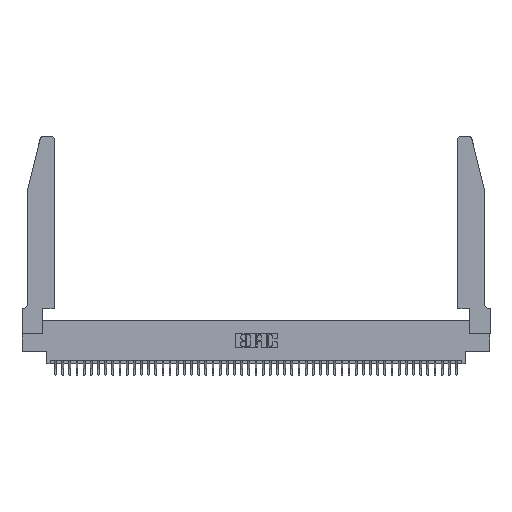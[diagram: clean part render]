
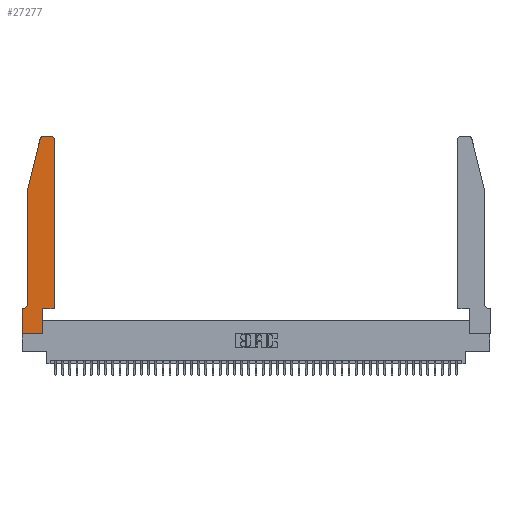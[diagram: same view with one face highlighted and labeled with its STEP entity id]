
A CAD part, top view. The second image highlights one B-rep face of the part: STEP entity #27277.
In plain terms, the highlighted planar face has unit normal (0, 0, 1).
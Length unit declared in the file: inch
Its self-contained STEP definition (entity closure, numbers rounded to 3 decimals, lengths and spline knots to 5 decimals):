
#20 = ORIENTED_EDGE ( 'NONE', *, *, #19385, .T. ) ;
#1429 = CARTESIAN_POINT ( 'NONE',  ( 0.4205, 2.75, 0.37 ) ) ;
#1964 = EDGE_CURVE ( 'NONE', #38628, #4420, #27230, .T. ) ;
#2141 = CARTESIAN_POINT ( 'NONE',  ( 0.4505, 0.35, 0.37 ) ) ;
#2412 = CARTESIAN_POINT ( 'NONE',  ( 0.2865, 0., 0.37 ) ) ;
#2573 = AXIS2_PLACEMENT_3D ( 'NONE', #45537, #16518, #23485 ) ;
#2690 = CARTESIAN_POINT ( 'NONE',  ( 0.0755, 2., 0.37 ) ) ;
#3716 = VECTOR ( 'NONE', #24638, 39.37008 ) ;
#3893 = EDGE_CURVE ( 'NONE', #40289, #14073, #43181, .T. ) ;
#4172 = CARTESIAN_POINT ( 'NONE',  ( 0.4505, 2.72, 0.37 ) ) ;
#4420 = VERTEX_POINT ( 'NONE', #40734 ) ;
#4967 = DIRECTION ( 'NONE',  ( 1., 0., 0. ) ) ;
#5245 = DIRECTION ( 'NONE',  ( 0., -1., 0. ) ) ;
#5766 = LINE ( 'NONE', #35948, #44447 ) ;
#6378 = ORIENTED_EDGE ( 'NONE', *, *, #39761, .T. ) ;
#6532 = LINE ( 'NONE', #11132, #37181 ) ;
#7448 = CARTESIAN_POINT ( 'NONE',  ( 0., 0.35, 0.37 ) ) ;
#8057 = VECTOR ( 'NONE', #4967, 39.37008 ) ;
#8680 = ORIENTED_EDGE ( 'NONE', *, *, #10243, .T. ) ;
#9904 = VECTOR ( 'NONE', #26915, 39.37008 ) ;
#10243 = EDGE_CURVE ( 'NONE', #4420, #34217, #5766, .T. ) ;
#11132 = CARTESIAN_POINT ( 'NONE',  ( 0.2605, 2.75, 0.37 ) ) ;
#11468 = LINE ( 'NONE', #28850, #13152 ) ;
#11727 = EDGE_CURVE ( 'NONE', #19697, #38628, #17912, .T. ) ;
#12339 = AXIS2_PLACEMENT_3D ( 'NONE', #13545, #38737, #16945 ) ;
#12400 = CARTESIAN_POINT ( 'NONE',  ( 0.284, 2.72, 0.37 ) ) ;
#13152 = VECTOR ( 'NONE', #43500, 39.37008 ) ;
#13545 = CARTESIAN_POINT ( 'NONE',  ( 0., 0.35, 0.37 ) ) ;
#14073 = VERTEX_POINT ( 'NONE', #34943 ) ;
#14181 = CIRCLE ( 'NONE', #2573, 0.03 ) ;
#14210 = ORIENTED_EDGE ( 'NONE', *, *, #1964, .T. ) ;
#15037 = EDGE_CURVE ( 'NONE', #43915, #40289, #6532, .T. ) ;
#16192 = CARTESIAN_POINT ( 'NONE',  ( 0.0755, 2., 0.37 ) ) ;
#16197 = ORIENTED_EDGE ( 'NONE', *, *, #16259, .T. ) ;
#16244 = CARTESIAN_POINT ( 'NONE',  ( 0.0055, 0.35, 0.37 ) ) ;
#16259 = EDGE_CURVE ( 'NONE', #32025, #25647, #35874, .T. ) ;
#16268 = FACE_OUTER_BOUND ( 'NONE', #31477, .T. ) ;
#16518 = DIRECTION ( 'NONE',  ( 0., 0., 1. ) ) ;
#16660 = ORIENTED_EDGE ( 'NONE', *, *, #27685, .T. ) ;
#16945 = DIRECTION ( 'NONE',  ( 1., 0., 0. ) ) ;
#17912 = LINE ( 'NONE', #45498, #8057 ) ;
#17932 = DIRECTION ( 'NONE',  ( -0.239, -0.971, 0. ) ) ;
#17935 = LINE ( 'NONE', #19531, #45042 ) ;
#18639 = CARTESIAN_POINT ( 'NONE',  ( 0.4505, 0.35, 0.37 ) ) ;
#19170 = VERTEX_POINT ( 'NONE', #4172 ) ;
#19385 = EDGE_CURVE ( 'NONE', #14073, #32025, #39925, .T. ) ;
#19394 = ORIENTED_EDGE ( 'NONE', *, *, #23281, .T. ) ;
#19478 = ORIENTED_EDGE ( 'NONE', *, *, #15037, .T. ) ;
#19531 = CARTESIAN_POINT ( 'NONE',  ( 0., 0., 0.37 ) ) ;
#19697 = VERTEX_POINT ( 'NONE', #34327 ) ;
#21006 = EDGE_CURVE ( 'NONE', #29517, #29905, #11468, .T. ) ;
#21138 = DIRECTION ( 'NONE',  ( 1., 0., 0. ) ) ;
#22261 = CIRCLE ( 'NONE', #24636, 0.07 ) ;
#23281 = EDGE_CURVE ( 'NONE', #19170, #43915, #14181, .T. ) ;
#23485 = DIRECTION ( 'NONE',  ( 1., 0., 0. ) ) ;
#24636 = AXIS2_PLACEMENT_3D ( 'NONE', #44563, #26358, #41343 ) ;
#24638 = DIRECTION ( 'NONE',  ( 0., 1., 0. ) ) ;
#25137 = EDGE_CURVE ( 'NONE', #25647, #29517, #22261, .T. ) ;
#25647 = VERTEX_POINT ( 'NONE', #43874 ) ;
#26358 = DIRECTION ( 'NONE',  ( 0., 0., -1. ) ) ;
#26915 = DIRECTION ( 'NONE',  ( 0., 1., 0. ) ) ;
#27230 = LINE ( 'NONE', #30787, #9904 ) ;
#27277 = ADVANCED_FACE ( 'NONE', ( #16268 ), #31794, .T. ) ;
#27685 = EDGE_CURVE ( 'NONE', #29905, #19697, #17935, .T. ) ;
#28850 = CARTESIAN_POINT ( 'NONE',  ( 0.0755, 0.35, 0.37 ) ) ;
#29517 = VERTEX_POINT ( 'NONE', #16244 ) ;
#29905 = VERTEX_POINT ( 'NONE', #7448 ) ;
#30787 = CARTESIAN_POINT ( 'NONE',  ( 0.2865, 0.35, 0.37 ) ) ;
#31257 = DIRECTION ( 'NONE',  ( 0., 0., 1. ) ) ;
#31477 = EDGE_LOOP ( 'NONE', ( #19478, #36845, #20, #16197, #43846, #43050, #16660, #35146, #14210, #8680, #6378, #19394 ) ) ;
#31794 = PLANE ( 'NONE',  #12339 ) ;
#32025 = VERTEX_POINT ( 'NONE', #16192 ) ;
#32424 = AXIS2_PLACEMENT_3D ( 'NONE', #12400, #31257, #38211 ) ;
#33981 = CARTESIAN_POINT ( 'NONE',  ( 0.284, 2.75, 0.37 ) ) ;
#34217 = VERTEX_POINT ( 'NONE', #18639 ) ;
#34327 = CARTESIAN_POINT ( 'NONE',  ( 0., 0., 0.37 ) ) ;
#34943 = CARTESIAN_POINT ( 'NONE',  ( 0.25487, 2.72718, 0.37 ) ) ;
#35146 = ORIENTED_EDGE ( 'NONE', *, *, #11727, .T. ) ;
#35874 = LINE ( 'NONE', #37155, #42215 ) ;
#35948 = CARTESIAN_POINT ( 'NONE',  ( 0.4505, 0.35, 0.37 ) ) ;
#36845 = ORIENTED_EDGE ( 'NONE', *, *, #3893, .T. ) ;
#37155 = CARTESIAN_POINT ( 'NONE',  ( 0.0755, 2., 0.37 ) ) ;
#37181 = VECTOR ( 'NONE', #41124, 39.37008 ) ;
#38211 = DIRECTION ( 'NONE',  ( 1., 0., 0. ) ) ;
#38628 = VERTEX_POINT ( 'NONE', #2412 ) ;
#38737 = DIRECTION ( 'NONE',  ( 0., 0., 1. ) ) ;
#39761 = EDGE_CURVE ( 'NONE', #34217, #19170, #44785, .T. ) ;
#39925 = LINE ( 'NONE', #2690, #41075 ) ;
#40222 = DIRECTION ( 'NONE',  ( 0., -1., 0. ) ) ;
#40289 = VERTEX_POINT ( 'NONE', #33981 ) ;
#40734 = CARTESIAN_POINT ( 'NONE',  ( 0.2865, 0.35, 0.37 ) ) ;
#41075 = VECTOR ( 'NONE', #17932, 39.37008 ) ;
#41124 = DIRECTION ( 'NONE',  ( -1., 0., 0. ) ) ;
#41343 = DIRECTION ( 'NONE',  ( -1., 0., 0. ) ) ;
#42215 = VECTOR ( 'NONE', #40222, 39.37008 ) ;
#43050 = ORIENTED_EDGE ( 'NONE', *, *, #21006, .T. ) ;
#43181 = CIRCLE ( 'NONE', #32424, 0.03 ) ;
#43500 = DIRECTION ( 'NONE',  ( -1., 0., 0. ) ) ;
#43846 = ORIENTED_EDGE ( 'NONE', *, *, #25137, .T. ) ;
#43874 = CARTESIAN_POINT ( 'NONE',  ( 0.0755, 0.42, 0.37 ) ) ;
#43915 = VERTEX_POINT ( 'NONE', #1429 ) ;
#44447 = VECTOR ( 'NONE', #21138, 39.37008 ) ;
#44563 = CARTESIAN_POINT ( 'NONE',  ( 0.0055, 0.42, 0.37 ) ) ;
#44785 = LINE ( 'NONE', #2141, #3716 ) ;
#45042 = VECTOR ( 'NONE', #5245, 39.37008 ) ;
#45498 = CARTESIAN_POINT ( 'NONE',  ( 0., 0., 0.37 ) ) ;
#45537 = CARTESIAN_POINT ( 'NONE',  ( 0.4205, 2.72, 0.37 ) ) ;
